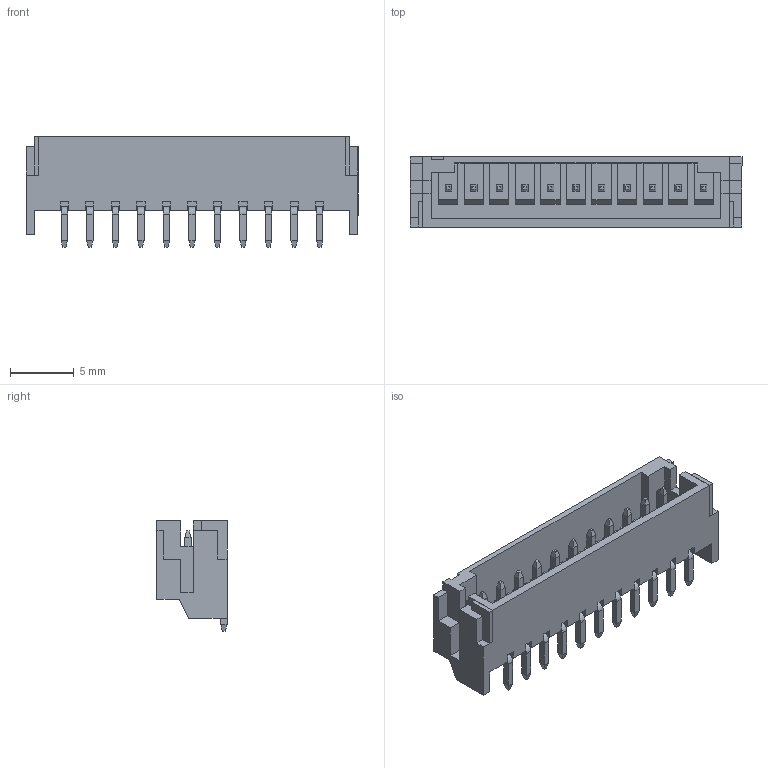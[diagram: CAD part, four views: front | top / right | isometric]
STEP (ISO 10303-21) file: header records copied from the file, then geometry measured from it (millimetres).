
FILE_DESCRIPTION (( 'STEP AP203' ), '1' );
FILE_NAME ('140-511-417-060.STEP', '2020-03-31T20:23:52', ( '' ), ( '' ), 'SwSTEP 2.0', 'SolidWorks 2016', '' );
FILE_SCHEMA (( 'CONFIG_CONTROL_DESIGN' ));
Length unit declared in the file: millimetre
Products named in the file (4): RA SMT Housing_511; RA SMT Contact; 140-511-417-060; RA SMT Pad
Assembly tree (14 placements, depth 2):
  140-511-417-060
    RA SMT Housing_511
    RA SMT Contact  x11
    RA SMT Pad  x2
Bounding box: 26 x 5.5 x 8.65 mm (x, y, z)
Volume: 350.9 mm3; surface area: 1328.3 mm2
Topology: 14 solids, 14 shells, 586 faces, 1420 edges, 858 vertices
Faces by surface type: plane 542, cylinder 44
Entity records: 9790 total; most frequent: CARTESIAN_POINT 1635, ORIENTED_EDGE 1616, DIRECTION 1410, EDGE_CURVE 808, LINE 800, VECTOR 800, VERTEX_POINT 530, AXIS2_PLACEMENT_3D 305
